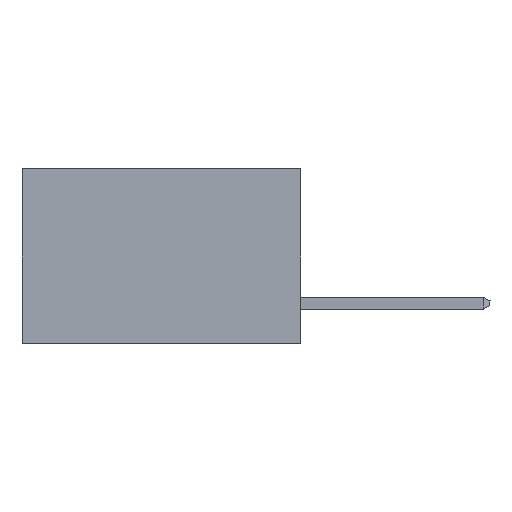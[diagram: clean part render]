
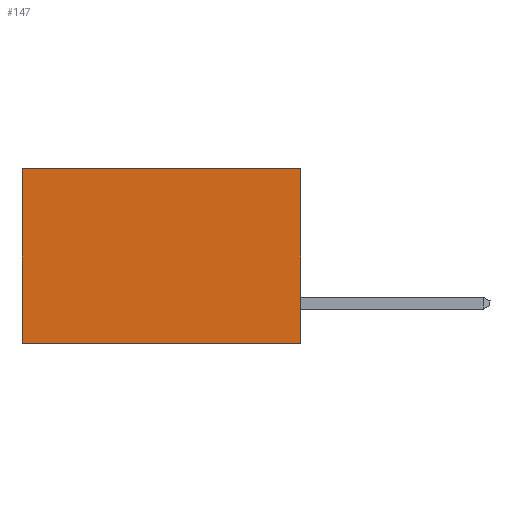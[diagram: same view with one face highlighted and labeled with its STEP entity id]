
A CAD part, left-side view. The second image highlights one B-rep face of the part: STEP entity #147.
In plain terms, the highlighted planar face has unit normal (-1, 0, 0).
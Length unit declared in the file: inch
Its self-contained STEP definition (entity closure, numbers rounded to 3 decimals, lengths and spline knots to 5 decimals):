
#147 = ADVANCED_FACE ( 'NONE', ( #9374 ), #9595, .F. ) ;
#696 = EDGE_CURVE ( 'NONE', #5824, #3729, #7936, .T. ) ;
#1551 = CARTESIAN_POINT ( 'NONE',  ( 0.277, 0., -0.37 ) ) ;
#1592 = VERTEX_POINT ( 'NONE', #5529 ) ;
#1685 = EDGE_LOOP ( 'NONE', ( #3171, #3193, #3203, #3227 ) ) ;
#2312 = DIRECTION ( 'NONE',  ( 0., 0., -1. ) ) ;
#3065 = CARTESIAN_POINT ( 'NONE',  ( 0.277, 0.59, -0.37 ) ) ;
#3069 = VECTOR ( 'NONE', #4308, 39.37008 ) ;
#3171 = ORIENTED_EDGE ( 'NONE', *, *, #6368, .T. ) ;
#3193 = ORIENTED_EDGE ( 'NONE', *, *, #3240, .F. ) ;
#3203 = ORIENTED_EDGE ( 'NONE', *, *, #3302, .F. ) ;
#3227 = ORIENTED_EDGE ( 'NONE', *, *, #696, .T. ) ;
#3233 = CARTESIAN_POINT ( 'NONE',  ( 0.277, 0., 0. ) ) ;
#3240 = EDGE_CURVE ( 'NONE', #4085, #1592, #4335, .T. ) ;
#3302 = EDGE_CURVE ( 'NONE', #5824, #4085, #3760, .T. ) ;
#3460 = VECTOR ( 'NONE', #9756, 39.37008 ) ;
#3509 = DIRECTION ( 'NONE',  ( 0., 0., -1. ) ) ;
#3729 = VERTEX_POINT ( 'NONE', #10961 ) ;
#3760 = LINE ( 'NONE', #1551, #3460 ) ;
#4085 = VERTEX_POINT ( 'NONE', #10187 ) ;
#4308 = DIRECTION ( 'NONE',  ( 0., 1., 0. ) ) ;
#4335 = LINE ( 'NONE', #7206, #10918 ) ;
#4855 = LINE ( 'NONE', #3065, #11366 ) ;
#5529 = CARTESIAN_POINT ( 'NONE',  ( 0.277, 0.59, -0.37 ) ) ;
#5655 = DIRECTION ( 'NONE',  ( 1., 0., 0. ) ) ;
#5824 = VERTEX_POINT ( 'NONE', #6365 ) ;
#6004 = CARTESIAN_POINT ( 'NONE',  ( 0.277, 0., -0.37 ) ) ;
#6365 = CARTESIAN_POINT ( 'NONE',  ( 0.277, 0., 0. ) ) ;
#6368 = EDGE_CURVE ( 'NONE', #3729, #1592, #4855, .T. ) ;
#7206 = CARTESIAN_POINT ( 'NONE',  ( 0.277, 0., -0.37 ) ) ;
#7936 = LINE ( 'NONE', #3233, #3069 ) ;
#9374 = FACE_OUTER_BOUND ( 'NONE', #1685, .T. ) ;
#9595 = PLANE ( 'NONE',  #10837 ) ;
#9756 = DIRECTION ( 'NONE',  ( 0., 0., -1. ) ) ;
#10187 = CARTESIAN_POINT ( 'NONE',  ( 0.277, 0., -0.37 ) ) ;
#10600 = DIRECTION ( 'NONE',  ( 0., 1., 0. ) ) ;
#10837 = AXIS2_PLACEMENT_3D ( 'NONE', #6004, #5655, #3509 ) ;
#10918 = VECTOR ( 'NONE', #10600, 39.37008 ) ;
#10961 = CARTESIAN_POINT ( 'NONE',  ( 0.277, 0.59, 0. ) ) ;
#11366 = VECTOR ( 'NONE', #2312, 39.37008 ) ;
